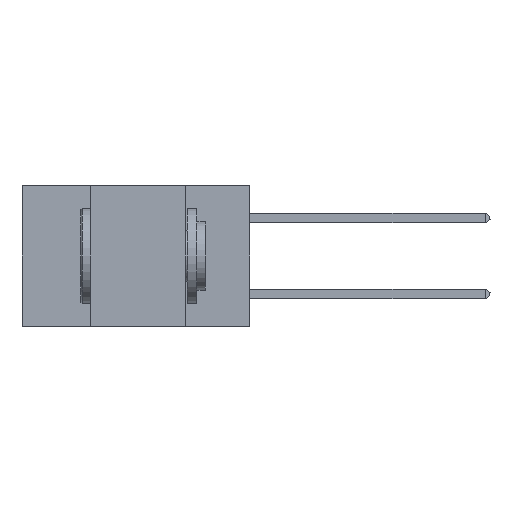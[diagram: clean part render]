
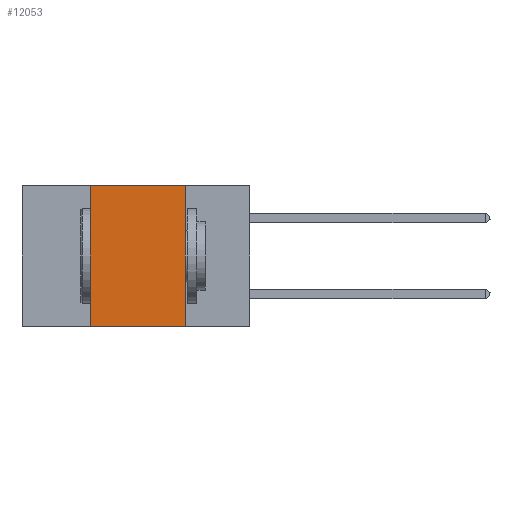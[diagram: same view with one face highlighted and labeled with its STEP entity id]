
A CAD part, left-side view. The second image highlights one B-rep face of the part: STEP entity #12053.
In plain terms, the highlighted planar face has unit normal (-1, 0, 0).
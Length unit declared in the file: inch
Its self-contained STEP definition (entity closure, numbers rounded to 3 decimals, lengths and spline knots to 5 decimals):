
#422 = CARTESIAN_POINT ( 'NONE',  ( 0., 0.6, 0. ) ) ;
#1455 = DIRECTION ( 'NONE',  ( 1., 0., 0. ) ) ;
#4239 = CARTESIAN_POINT ( 'NONE',  ( 0., 0.6, 0. ) ) ;
#6053 = CARTESIAN_POINT ( 'NONE',  ( 0., 0.42, 0. ) ) ;
#7274 = VECTOR ( 'NONE', #33115, 39.37008 ) ;
#9325 = CARTESIAN_POINT ( 'NONE',  ( 0., 0.6, -0.37 ) ) ;
#10685 = VERTEX_POINT ( 'NONE', #28517 ) ;
#11096 = ORIENTED_EDGE ( 'NONE', *, *, #32340, .F. ) ;
#12053 = ADVANCED_FACE ( 'NONE', ( #31914 ), #25570, .F. ) ;
#12233 = DIRECTION ( 'NONE',  ( 0., -1., 0. ) ) ;
#14757 = CARTESIAN_POINT ( 'NONE',  ( 0., 0.17, 0. ) ) ;
#15328 = CARTESIAN_POINT ( 'NONE',  ( 0., 0.17, 0. ) ) ;
#15943 = LINE ( 'NONE', #9325, #19693 ) ;
#17393 = ORIENTED_EDGE ( 'NONE', *, *, #28365, .T. ) ;
#18448 = AXIS2_PLACEMENT_3D ( 'NONE', #4239, #1455, #22386 ) ;
#19693 = VECTOR ( 'NONE', #12233, 39.37008 ) ;
#22386 = DIRECTION ( 'NONE',  ( 0., 0., -1. ) ) ;
#23146 = VERTEX_POINT ( 'NONE', #37260 ) ;
#24517 = DIRECTION ( 'NONE',  ( 0., -1., 0. ) ) ;
#25069 = LINE ( 'NONE', #6053, #36342 ) ;
#25570 = PLANE ( 'NONE',  #18448 ) ;
#26333 = CARTESIAN_POINT ( 'NONE',  ( 0., 0.42, -0.37 ) ) ;
#26519 = EDGE_CURVE ( 'NONE', #23146, #38948, #28298, .T. ) ;
#26997 = DIRECTION ( 'NONE',  ( 0., 0., 1. ) ) ;
#27013 = VERTEX_POINT ( 'NONE', #26333 ) ;
#28298 = LINE ( 'NONE', #422, #29720 ) ;
#28365 = EDGE_CURVE ( 'NONE', #27013, #10685, #15943, .T. ) ;
#28517 = CARTESIAN_POINT ( 'NONE',  ( 0., 0.17, -0.37 ) ) ;
#29720 = VECTOR ( 'NONE', #24517, 39.37008 ) ;
#31130 = EDGE_LOOP ( 'NONE', ( #33061, #33372, #11096, #17393 ) ) ;
#31914 = FACE_OUTER_BOUND ( 'NONE', #31130, .T. ) ;
#32340 = EDGE_CURVE ( 'NONE', #27013, #23146, #25069, .T. ) ;
#33061 = ORIENTED_EDGE ( 'NONE', *, *, #36338, .F. ) ;
#33115 = DIRECTION ( 'NONE',  ( 0., 0., -1. ) ) ;
#33372 = ORIENTED_EDGE ( 'NONE', *, *, #26519, .F. ) ;
#36338 = EDGE_CURVE ( 'NONE', #38948, #10685, #36502, .T. ) ;
#36342 = VECTOR ( 'NONE', #26997, 39.37008 ) ;
#36502 = LINE ( 'NONE', #14757, #7274 ) ;
#37260 = CARTESIAN_POINT ( 'NONE',  ( 0., 0.42, 0. ) ) ;
#38948 = VERTEX_POINT ( 'NONE', #15328 ) ;
